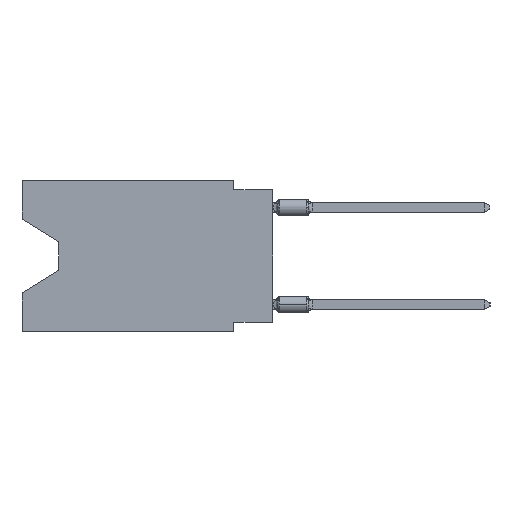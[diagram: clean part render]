
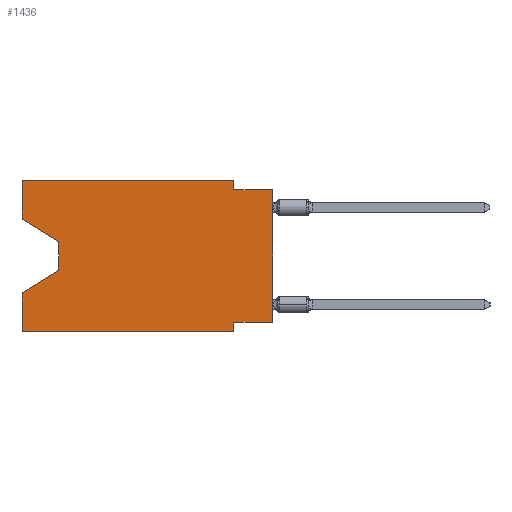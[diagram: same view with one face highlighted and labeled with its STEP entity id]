
A CAD part, left-side view. The second image highlights one B-rep face of the part: STEP entity #1436.
In plain terms, the highlighted planar face has unit normal (-1, 0, 0).
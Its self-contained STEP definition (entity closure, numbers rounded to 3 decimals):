
#124 = ORIENTED_EDGE ( 'NONE', *, *, #27002, .T. ) ;
#708 = ORIENTED_EDGE ( 'NONE', *, *, #23912, .F. ) ;
#801 = CARTESIAN_POINT ( 'NONE',  ( 0., 16.383, 0. ) ) ;
#1436 = ADVANCED_FACE ( 'NONE', ( #4924 ), #2092, .F. ) ;
#1698 = AXIS2_PLACEMENT_3D ( 'NONE', #13661, #4625, #28016 ) ;
#1791 = CARTESIAN_POINT ( 'NONE',  ( 0., 2.54, 0. ) ) ;
#2092 = PLANE ( 'NONE',  #1698 ) ;
#2294 = VECTOR ( 'NONE', #15614, 1000. ) ;
#2793 = VERTEX_POINT ( 'NONE', #21217 ) ;
#3367 = VECTOR ( 'NONE', #24531, 1000. ) ;
#3637 = EDGE_CURVE ( 'NONE', #22702, #11203, #24934, .T. ) ;
#4286 = CARTESIAN_POINT ( 'NONE',  ( 0., 13.97, -4.013 ) ) ;
#4625 = DIRECTION ( 'NONE',  ( 1., 0., 0. ) ) ;
#4635 = VECTOR ( 'NONE', #14046, 1000. ) ;
#4924 = FACE_OUTER_BOUND ( 'NONE', #27241, .T. ) ;
#5021 = CARTESIAN_POINT ( 'NONE',  ( 0., 16.383, -2.546 ) ) ;
#5250 = VECTOR ( 'NONE', #26337, 1000. ) ;
#5256 = CARTESIAN_POINT ( 'NONE',  ( 0., 2.54, -9.271 ) ) ;
#5357 = CARTESIAN_POINT ( 'NONE',  ( 0., 16.383, -2.546 ) ) ;
#5731 = VECTOR ( 'NONE', #20325, 1000. ) ;
#5760 = CARTESIAN_POINT ( 'NONE',  ( 0., 16.383, -9.906 ) ) ;
#6477 = ORIENTED_EDGE ( 'NONE', *, *, #10070, .T. ) ;
#6637 = VERTEX_POINT ( 'NONE', #15459 ) ;
#6694 = DIRECTION ( 'NONE',  ( 0., 0., -1. ) ) ;
#6746 = ORIENTED_EDGE ( 'NONE', *, *, #26639, .F. ) ;
#7095 = CARTESIAN_POINT ( 'NONE',  ( 0., 2.54, -9.906 ) ) ;
#7740 = CARTESIAN_POINT ( 'NONE',  ( 0., 0., -9.271 ) ) ;
#8034 = DIRECTION ( 'NONE',  ( 0., -1., 0. ) ) ;
#8104 = CARTESIAN_POINT ( 'NONE',  ( 0., 0., 0. ) ) ;
#8203 = ORIENTED_EDGE ( 'NONE', *, *, #29283, .T. ) ;
#8408 = VERTEX_POINT ( 'NONE', #7740 ) ;
#8544 = EDGE_CURVE ( 'NONE', #6637, #2793, #17806, .T. ) ;
#9149 = VERTEX_POINT ( 'NONE', #5021 ) ;
#9672 = CARTESIAN_POINT ( 'NONE',  ( 0., 0., -0.635 ) ) ;
#10070 = EDGE_CURVE ( 'NONE', #11203, #17369, #29055, .T. ) ;
#10338 = LINE ( 'NONE', #5357, #29473 ) ;
#10734 = LINE ( 'NONE', #5760, #29158 ) ;
#10964 = VECTOR ( 'NONE', #6694, 1000. ) ;
#11142 = LINE ( 'NONE', #17756, #5731 ) ;
#11185 = CARTESIAN_POINT ( 'NONE',  ( 0., 0., -0.635 ) ) ;
#11203 = VERTEX_POINT ( 'NONE', #19133 ) ;
#11243 = CARTESIAN_POINT ( 'NONE',  ( 0., 2.54, -0.635 ) ) ;
#12676 = VERTEX_POINT ( 'NONE', #28022 ) ;
#12698 = VERTEX_POINT ( 'NONE', #11243 ) ;
#12892 = CARTESIAN_POINT ( 'NONE',  ( 0., 13.97, -5.893 ) ) ;
#13225 = LINE ( 'NONE', #801, #28137 ) ;
#13661 = CARTESIAN_POINT ( 'NONE',  ( 0., 16.383, 0. ) ) ;
#14046 = DIRECTION ( 'NONE',  ( 0., 1., 0. ) ) ;
#14152 = LINE ( 'NONE', #7095, #21938 ) ;
#14710 = LINE ( 'NONE', #8104, #5250 ) ;
#15181 = EDGE_CURVE ( 'NONE', #2793, #12698, #29082, .T. ) ;
#15459 = CARTESIAN_POINT ( 'NONE',  ( 0., 16.383, 0. ) ) ;
#15543 = ORIENTED_EDGE ( 'NONE', *, *, #17081, .F. ) ;
#15614 = DIRECTION ( 'NONE',  ( 0., 0.855, -0.519 ) ) ;
#15806 = ORIENTED_EDGE ( 'NONE', *, *, #15181, .F. ) ;
#17081 = EDGE_CURVE ( 'NONE', #8408, #25374, #21308, .T. ) ;
#17098 = DIRECTION ( 'NONE',  ( 0., -0.855, -0.519 ) ) ;
#17168 = ORIENTED_EDGE ( 'NONE', *, *, #23805, .T. ) ;
#17369 = VERTEX_POINT ( 'NONE', #26878 ) ;
#17498 = VERTEX_POINT ( 'NONE', #9672 ) ;
#17756 = CARTESIAN_POINT ( 'NONE',  ( 0., 16.383, 0. ) ) ;
#17806 = LINE ( 'NONE', #24435, #25870 ) ;
#17981 = CARTESIAN_POINT ( 'NONE',  ( 0., 16.383, -9.906 ) ) ;
#18204 = CARTESIAN_POINT ( 'NONE',  ( 0., 13.97, -4.013 ) ) ;
#18506 = ORIENTED_EDGE ( 'NONE', *, *, #3637, .T. ) ;
#19133 = CARTESIAN_POINT ( 'NONE',  ( 0., 13.97, -5.893 ) ) ;
#20325 = DIRECTION ( 'NONE',  ( 0., 0., 1. ) ) ;
#21217 = CARTESIAN_POINT ( 'NONE',  ( 0., 2.54, 0. ) ) ;
#21258 = DIRECTION ( 'NONE',  ( 0., 0., -1. ) ) ;
#21308 = LINE ( 'NONE', #25979, #4635 ) ;
#21938 = VECTOR ( 'NONE', #21258, 1000. ) ;
#22255 = VERTEX_POINT ( 'NONE', #17981 ) ;
#22448 = DIRECTION ( 'NONE',  ( 0., 0., 1. ) ) ;
#22572 = EDGE_CURVE ( 'NONE', #22255, #17369, #13225, .T. ) ;
#22702 = VERTEX_POINT ( 'NONE', #18204 ) ;
#23236 = ORIENTED_EDGE ( 'NONE', *, *, #8544, .F. ) ;
#23501 = ORIENTED_EDGE ( 'NONE', *, *, #24010, .F. ) ;
#23805 = EDGE_CURVE ( 'NONE', #22255, #12676, #10734, .T. ) ;
#23912 = EDGE_CURVE ( 'NONE', #12698, #17498, #29453, .T. ) ;
#24010 = EDGE_CURVE ( 'NONE', #25374, #12676, #14152, .T. ) ;
#24435 = CARTESIAN_POINT ( 'NONE',  ( 0., 16.383, 0. ) ) ;
#24531 = DIRECTION ( 'NONE',  ( 0., 0., -1. ) ) ;
#24934 = LINE ( 'NONE', #4286, #10964 ) ;
#25374 = VERTEX_POINT ( 'NONE', #5256 ) ;
#25780 = VECTOR ( 'NONE', #29138, 1000. ) ;
#25870 = VECTOR ( 'NONE', #27318, 1000. ) ;
#25979 = CARTESIAN_POINT ( 'NONE',  ( 0., 0., -9.271 ) ) ;
#26337 = DIRECTION ( 'NONE',  ( 0., 0., 1. ) ) ;
#26639 = EDGE_CURVE ( 'NONE', #9149, #6637, #11142, .T. ) ;
#26878 = CARTESIAN_POINT ( 'NONE',  ( 0., 16.383, -7.36 ) ) ;
#27002 = EDGE_CURVE ( 'NONE', #8408, #17498, #14710, .T. ) ;
#27241 = EDGE_LOOP ( 'NONE', ( #8203, #18506, #6477, #27394, #17168, #23501, #15543, #124, #708, #15806, #23236, #6746 ) ) ;
#27318 = DIRECTION ( 'NONE',  ( 0., -1., 0. ) ) ;
#27394 = ORIENTED_EDGE ( 'NONE', *, *, #22572, .F. ) ;
#28016 = DIRECTION ( 'NONE',  ( 0., 0., -1. ) ) ;
#28022 = CARTESIAN_POINT ( 'NONE',  ( 0., 2.54, -9.906 ) ) ;
#28137 = VECTOR ( 'NONE', #22448, 1000. ) ;
#29055 = LINE ( 'NONE', #12892, #2294 ) ;
#29082 = LINE ( 'NONE', #1791, #3367 ) ;
#29138 = DIRECTION ( 'NONE',  ( 0., -1., 0. ) ) ;
#29158 = VECTOR ( 'NONE', #8034, 1000. ) ;
#29283 = EDGE_CURVE ( 'NONE', #9149, #22702, #10338, .T. ) ;
#29453 = LINE ( 'NONE', #11185, #25780 ) ;
#29473 = VECTOR ( 'NONE', #17098, 1000. ) ;
